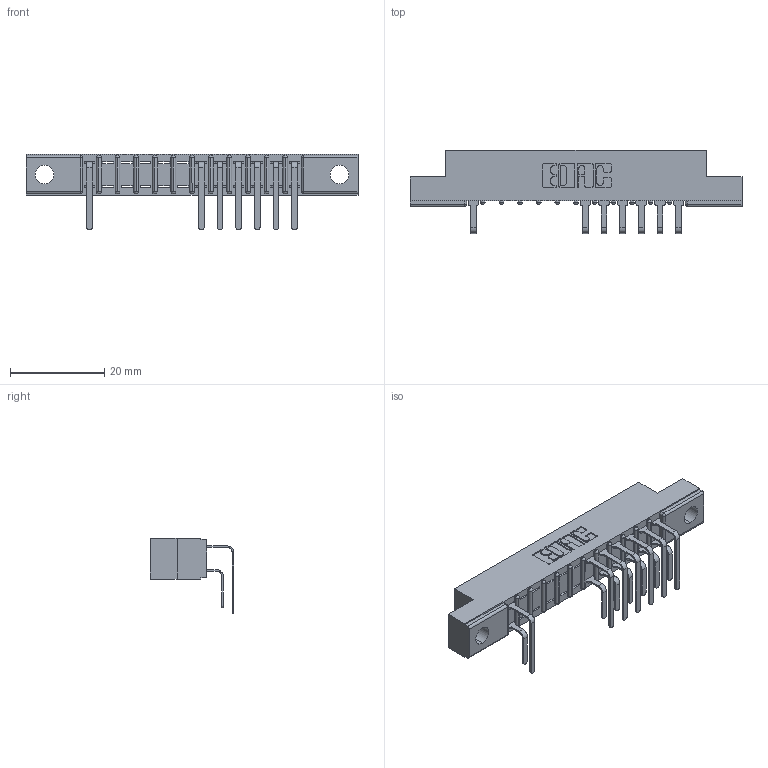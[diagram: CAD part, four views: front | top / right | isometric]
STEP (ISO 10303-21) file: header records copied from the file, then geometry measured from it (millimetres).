
FILE_DESCRIPTION (( 'STEP AP203' ), '1' );
FILE_NAME ('307-012-559-102.STEP', '2018-08-02T22:34:02', ( '' ), ( '' ), 'SwSTEP 2.0', 'SolidWorks 2016', '' );
FILE_SCHEMA (( 'CONFIG_CONTROL_DESIGN' ));
Length unit declared in the file: inch
Products named in the file (4): 307 Part_.128 Dia Mounting Holes; 307-290-001_558 559 - 1 (Single); 307-290-001_559 - 2 (Single); 307-012-559-102
Assembly tree (15 placements, depth 2):
  307-012-559-102
    307 Part_.128 Dia Mounting Holes
    307-290-001_558 559 - 1 (Single)  x7
    307-290-001_559 - 2 (Single)  x7
Bounding box: 70.56 x 17.69 x 16.08 mm (x, y, z)
Volume: 4461.3 mm3; surface area: 6789.9 mm2
Topology: 15 solids, 15 shells, 931 faces, 2631 edges, 1698 vertices
Faces by surface type: plane 592, cylinder 313, sphere 26
Entity records: 15499 total; most frequent: CARTESIAN_POINT 2588, ORIENTED_EDGE 2570, DIRECTION 2537, EDGE_CURVE 1285, LINE 971, VECTOR 971, VERTEX_POINT 834, AXIS2_PLACEMENT_3D 783
